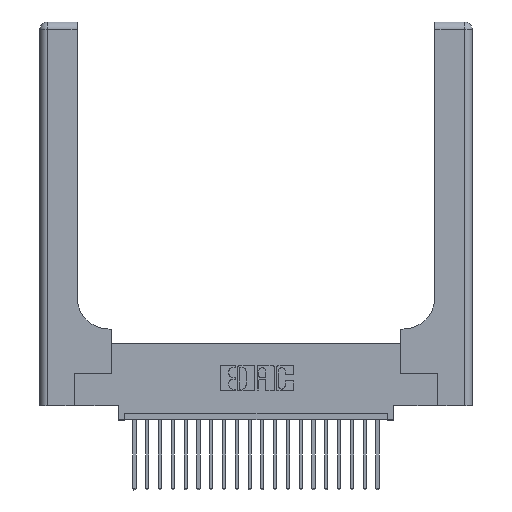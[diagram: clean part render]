
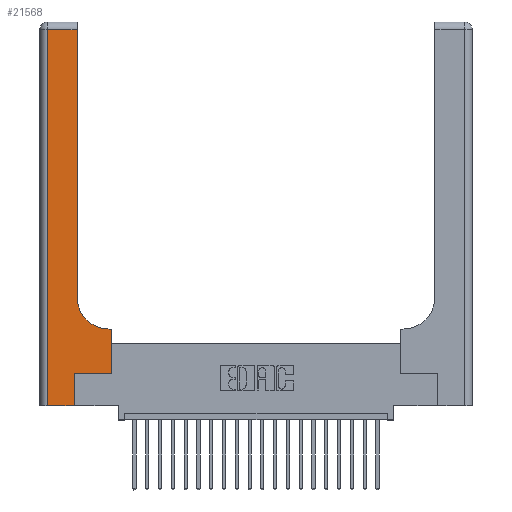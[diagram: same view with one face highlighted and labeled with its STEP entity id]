
A CAD part, top view. The second image highlights one B-rep face of the part: STEP entity #21568.
In plain terms, the highlighted planar face has unit normal (0, 0, 1).
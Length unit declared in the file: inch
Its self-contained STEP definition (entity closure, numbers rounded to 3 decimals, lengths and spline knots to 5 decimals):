
#398 = DIRECTION ( 'NONE',  ( -1., 0., 0. ) ) ;
#539 = ORIENTED_EDGE ( 'NONE', *, *, #11765, .T. ) ;
#721 = LINE ( 'NONE', #16037, #9227 ) ;
#843 = VERTEX_POINT ( 'NONE', #20886 ) ;
#1010 = VECTOR ( 'NONE', #8864, 39.37008 ) ;
#1821 = ORIENTED_EDGE ( 'NONE', *, *, #8021, .T. ) ;
#2316 = VECTOR ( 'NONE', #19086, 39.37008 ) ;
#2459 = VERTEX_POINT ( 'NONE', #20479 ) ;
#2486 = DIRECTION ( 'NONE',  ( 0., 0., -1. ) ) ;
#3061 = ORIENTED_EDGE ( 'NONE', *, *, #8274, .T. ) ;
#3095 = VERTEX_POINT ( 'NONE', #4897 ) ;
#3193 = EDGE_CURVE ( 'NONE', #3095, #19345, #721, .T. ) ;
#3283 = DIRECTION ( 'NONE',  ( -1., 0., 0. ) ) ;
#3541 = ORIENTED_EDGE ( 'NONE', *, *, #21443, .T. ) ;
#4176 = LINE ( 'NONE', #16125, #1010 ) ;
#4311 = DIRECTION ( 'NONE',  ( 1., 0., 0. ) ) ;
#4571 = LINE ( 'NONE', #12251, #6567 ) ;
#4684 = VERTEX_POINT ( 'NONE', #14455 ) ;
#4857 = VERTEX_POINT ( 'NONE', #11459 ) ;
#4897 = CARTESIAN_POINT ( 'NONE',  ( 0.269, 0.25, 0.37 ) ) ;
#4916 = VERTEX_POINT ( 'NONE', #23148 ) ;
#5070 = DIRECTION ( 'NONE',  ( 0., -1., 0. ) ) ;
#5210 = DIRECTION ( 'NONE',  ( 1., 0., 0. ) ) ;
#5370 = PLANE ( 'NONE',  #13407 ) ;
#5836 = VECTOR ( 'NONE', #20025, 39.37008 ) ;
#5901 = FACE_OUTER_BOUND ( 'NONE', #14107, .T. ) ;
#6567 = VECTOR ( 'NONE', #5070, 39.37008 ) ;
#7408 = VECTOR ( 'NONE', #3283, 39.37008 ) ;
#7472 = CARTESIAN_POINT ( 'NONE',  ( 0.5585, 0.25, 0.37 ) ) ;
#7503 = CARTESIAN_POINT ( 'NONE',  ( 0.2915, 0.85, 0.37 ) ) ;
#7574 = CARTESIAN_POINT ( 'NONE',  ( 0.5585, 0.25, 0.37 ) ) ;
#8021 = EDGE_CURVE ( 'NONE', #19345, #8381, #17140, .T. ) ;
#8274 = EDGE_CURVE ( 'NONE', #19827, #2459, #4176, .T. ) ;
#8381 = VERTEX_POINT ( 'NONE', #18145 ) ;
#8810 = ORIENTED_EDGE ( 'NONE', *, *, #11559, .T. ) ;
#8864 = DIRECTION ( 'NONE',  ( 0., 1., 0. ) ) ;
#9064 = LINE ( 'NONE', #19163, #2316 ) ;
#9227 = VECTOR ( 'NONE', #19452, 39.37008 ) ;
#9668 = CARTESIAN_POINT ( 'NONE',  ( 0.5415, 0.85, 0.37 ) ) ;
#11459 = CARTESIAN_POINT ( 'NONE',  ( 0.06, 2.94, 0.37 ) ) ;
#11559 = EDGE_CURVE ( 'NONE', #4857, #843, #4571, .T. ) ;
#11650 = ORIENTED_EDGE ( 'NONE', *, *, #3193, .T. ) ;
#11765 = EDGE_CURVE ( 'NONE', #2459, #4857, #21122, .T. ) ;
#12096 = EDGE_CURVE ( 'NONE', #4684, #3095, #9064, .T. ) ;
#12251 = CARTESIAN_POINT ( 'NONE',  ( 0.06, 3., 0.37 ) ) ;
#12558 = CARTESIAN_POINT ( 'NONE',  ( 0., 3., 0.37 ) ) ;
#12969 = VECTOR ( 'NONE', #5210, 39.37008 ) ;
#13038 = DIRECTION ( 'NONE',  ( 0., 0., -1. ) ) ;
#13407 = AXIS2_PLACEMENT_3D ( 'NONE', #12558, #13038, #17947 ) ;
#13738 = EDGE_CURVE ( 'NONE', #4916, #19827, #16654, .T. ) ;
#14107 = EDGE_LOOP ( 'NONE', ( #3061, #539, #8810, #3541, #17004, #11650, #1821, #17225, #21650 ) ) ;
#14117 = CARTESIAN_POINT ( 'NONE',  ( 0., 2.94, 0.37 ) ) ;
#14455 = CARTESIAN_POINT ( 'NONE',  ( 0.269, 0., 0.37 ) ) ;
#14872 = AXIS2_PLACEMENT_3D ( 'NONE', #9668, #2486, #4311 ) ;
#15800 = VECTOR ( 'NONE', #398, 39.37008 ) ;
#16037 = CARTESIAN_POINT ( 'NONE',  ( 0.269, 0.25, 0.37 ) ) ;
#16125 = CARTESIAN_POINT ( 'NONE',  ( 0.2915, 3., 0.37 ) ) ;
#16654 = CIRCLE ( 'NONE', #14872, 0.25 ) ;
#16793 = EDGE_CURVE ( 'NONE', #8381, #4916, #21089, .T. ) ;
#17004 = ORIENTED_EDGE ( 'NONE', *, *, #12096, .T. ) ;
#17140 = LINE ( 'NONE', #7472, #5836 ) ;
#17225 = ORIENTED_EDGE ( 'NONE', *, *, #16793, .T. ) ;
#17640 = CARTESIAN_POINT ( 'NONE',  ( 0., 0., 0.37 ) ) ;
#17947 = DIRECTION ( 'NONE',  ( -1., 0., 0. ) ) ;
#18145 = CARTESIAN_POINT ( 'NONE',  ( 0.5585, 0.6, 0.37 ) ) ;
#18836 = LINE ( 'NONE', #17640, #12969 ) ;
#19086 = DIRECTION ( 'NONE',  ( 0., 1., 0. ) ) ;
#19163 = CARTESIAN_POINT ( 'NONE',  ( 0.269, 0., 0.37 ) ) ;
#19345 = VERTEX_POINT ( 'NONE', #7574 ) ;
#19452 = DIRECTION ( 'NONE',  ( 1., 0., 0. ) ) ;
#19827 = VERTEX_POINT ( 'NONE', #7503 ) ;
#20025 = DIRECTION ( 'NONE',  ( 0., 1., 0. ) ) ;
#20479 = CARTESIAN_POINT ( 'NONE',  ( 0.2915, 2.94, 0.37 ) ) ;
#20886 = CARTESIAN_POINT ( 'NONE',  ( 0.06, 0., 0.37 ) ) ;
#21089 = LINE ( 'NONE', #21557, #15800 ) ;
#21122 = LINE ( 'NONE', #14117, #7408 ) ;
#21443 = EDGE_CURVE ( 'NONE', #843, #4684, #18836, .T. ) ;
#21557 = CARTESIAN_POINT ( 'NONE',  ( 0.2915, 0.6, 0.37 ) ) ;
#21568 = ADVANCED_FACE ( 'NONE', ( #5901 ), #5370, .F. ) ;
#21650 = ORIENTED_EDGE ( 'NONE', *, *, #13738, .T. ) ;
#23148 = CARTESIAN_POINT ( 'NONE',  ( 0.5415, 0.6, 0.37 ) ) ;
